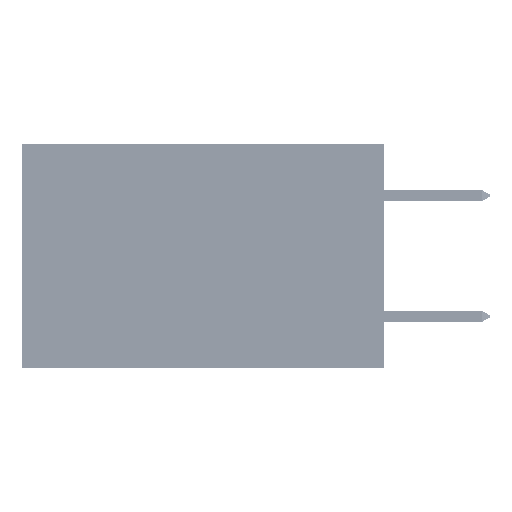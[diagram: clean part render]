
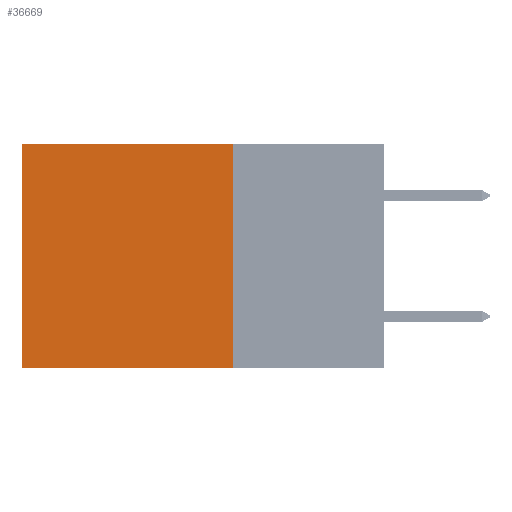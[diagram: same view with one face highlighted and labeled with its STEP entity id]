
A CAD part, left-side view. The second image highlights one B-rep face of the part: STEP entity #36669.
In plain terms, the highlighted planar face has unit normal (-1, 0, 0).
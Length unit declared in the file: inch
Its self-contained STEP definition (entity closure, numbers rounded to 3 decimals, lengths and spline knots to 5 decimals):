
#2014 = CARTESIAN_POINT ( 'NONE',  ( 0.2875, 0.25, -0.37 ) ) ;
#2636 = CARTESIAN_POINT ( 'NONE',  ( 0.2875, 0.25, 0. ) ) ;
#3728 = CARTESIAN_POINT ( 'NONE',  ( 0.2875, 0.6, 0. ) ) ;
#4660 = VECTOR ( 'NONE', #34589, 39.37008 ) ;
#5690 = FACE_OUTER_BOUND ( 'NONE', #35241, .T. ) ;
#6179 = ORIENTED_EDGE ( 'NONE', *, *, #30018, .F. ) ;
#7893 = VECTOR ( 'NONE', #37183, 39.37008 ) ;
#12498 = ORIENTED_EDGE ( 'NONE', *, *, #24107, .T. ) ;
#13113 = CARTESIAN_POINT ( 'NONE',  ( 0.2875, 0.25, -0.37 ) ) ;
#13640 = LINE ( 'NONE', #41958, #7893 ) ;
#18716 = VERTEX_POINT ( 'NONE', #23766 ) ;
#19232 = EDGE_CURVE ( 'NONE', #37816, #44218, #25518, .T. ) ;
#20617 = PLANE ( 'NONE',  #40757 ) ;
#23766 = CARTESIAN_POINT ( 'NONE',  ( 0.2875, 0.6, -0.37 ) ) ;
#24107 = EDGE_CURVE ( 'NONE', #44218, #18716, #38750, .T. ) ;
#25424 = VERTEX_POINT ( 'NONE', #13113 ) ;
#25518 = LINE ( 'NONE', #29477, #37570 ) ;
#25828 = DIRECTION ( 'NONE',  ( 1., 0., 0. ) ) ;
#26298 = CARTESIAN_POINT ( 'NONE',  ( 0.2875, 0.6, 0. ) ) ;
#27226 = EDGE_CURVE ( 'NONE', #37816, #25424, #13640, .T. ) ;
#29477 = CARTESIAN_POINT ( 'NONE',  ( 0.2875, 0.25, 0. ) ) ;
#30018 = EDGE_CURVE ( 'NONE', #25424, #18716, #46566, .T. ) ;
#32267 = DIRECTION ( 'NONE',  ( 0., 0., -1. ) ) ;
#32920 = DIRECTION ( 'NONE',  ( 0., 1., 0. ) ) ;
#34589 = DIRECTION ( 'NONE',  ( 0., 1., 0. ) ) ;
#35241 = EDGE_LOOP ( 'NONE', ( #12498, #6179, #35612, #40007 ) ) ;
#35612 = ORIENTED_EDGE ( 'NONE', *, *, #27226, .F. ) ;
#36669 = ADVANCED_FACE ( 'NONE', ( #5690 ), #20617, .F. ) ;
#37183 = DIRECTION ( 'NONE',  ( 0., 0., -1. ) ) ;
#37570 = VECTOR ( 'NONE', #32920, 39.37008 ) ;
#37816 = VERTEX_POINT ( 'NONE', #2636 ) ;
#38484 = DIRECTION ( 'NONE',  ( 0., 0., -1. ) ) ;
#38750 = LINE ( 'NONE', #26298, #40770 ) ;
#40007 = ORIENTED_EDGE ( 'NONE', *, *, #19232, .T. ) ;
#40757 = AXIS2_PLACEMENT_3D ( 'NONE', #41732, #25828, #32267 ) ;
#40770 = VECTOR ( 'NONE', #38484, 39.37008 ) ;
#41732 = CARTESIAN_POINT ( 'NONE',  ( 0.2875, 0.25, 0. ) ) ;
#41958 = CARTESIAN_POINT ( 'NONE',  ( 0.2875, 0.25, 0. ) ) ;
#44218 = VERTEX_POINT ( 'NONE', #3728 ) ;
#46566 = LINE ( 'NONE', #2014, #4660 ) ;
